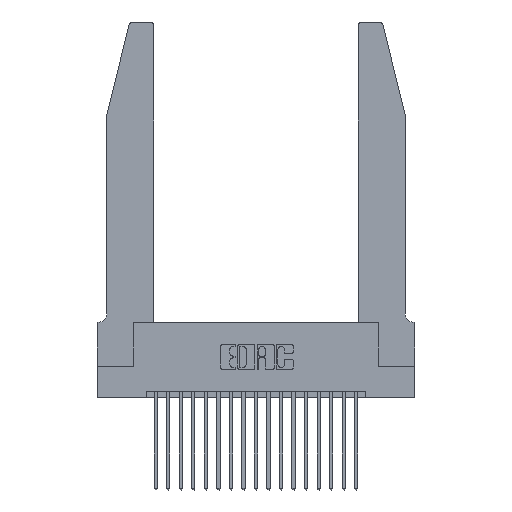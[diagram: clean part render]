
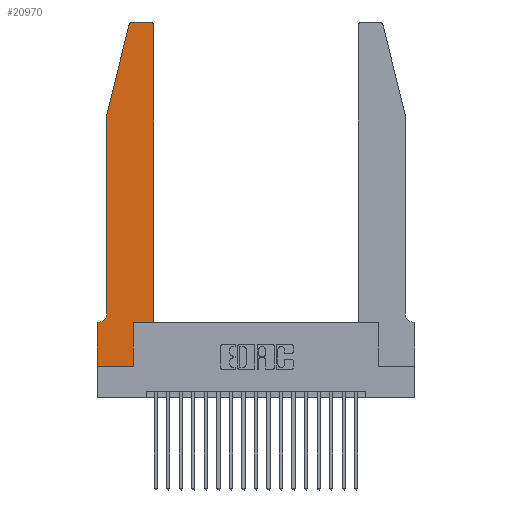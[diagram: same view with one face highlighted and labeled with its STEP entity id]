
A CAD part, top view. The second image highlights one B-rep face of the part: STEP entity #20970.
In plain terms, the highlighted planar face has unit normal (0, 0, 1).
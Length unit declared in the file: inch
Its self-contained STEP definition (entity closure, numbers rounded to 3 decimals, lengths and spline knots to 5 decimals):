
#87 = CARTESIAN_POINT ( 'NONE',  ( 0., 0.35, 0.37 ) ) ;
#249 = LINE ( 'NONE', #2413, #17041 ) ;
#292 = LINE ( 'NONE', #5435, #5316 ) ;
#384 = ORIENTED_EDGE ( 'NONE', *, *, #6104, .T. ) ;
#533 = DIRECTION ( 'NONE',  ( 0., 0., 1. ) ) ;
#713 = VERTEX_POINT ( 'NONE', #17654 ) ;
#732 = EDGE_CURVE ( 'NONE', #21065, #713, #19488, .T. ) ;
#775 = CARTESIAN_POINT ( 'NONE',  ( 0.25487, 2.72718, 0.37 ) ) ;
#1139 = ORIENTED_EDGE ( 'NONE', *, *, #11980, .T. ) ;
#1290 = CARTESIAN_POINT ( 'NONE',  ( 0.0755, 0.35, 0.37 ) ) ;
#1472 = LINE ( 'NONE', #15366, #5440 ) ;
#1486 = CARTESIAN_POINT ( 'NONE',  ( 0.0755, 2., 0.37 ) ) ;
#1848 = VECTOR ( 'NONE', #5260, 39.37008 ) ;
#2008 = CARTESIAN_POINT ( 'NONE',  ( 0., 0.35, 0.37 ) ) ;
#2413 = CARTESIAN_POINT ( 'NONE',  ( 0.4505, 0.35, 0.37 ) ) ;
#3207 = VECTOR ( 'NONE', #8109, 39.37008 ) ;
#3265 = VECTOR ( 'NONE', #12227, 39.37008 ) ;
#3444 = EDGE_LOOP ( 'NONE', ( #13576, #13081, #15457, #16988, #384, #16514, #11763, #8634, #13420, #1139, #20366, #21364 ) ) ;
#3725 = LINE ( 'NONE', #16472, #3207 ) ;
#3901 = EDGE_CURVE ( 'NONE', #11620, #21172, #4140, .T. ) ;
#4140 = LINE ( 'NONE', #1486, #12067 ) ;
#4184 = VERTEX_POINT ( 'NONE', #9055 ) ;
#4361 = VECTOR ( 'NONE', #16434, 39.37008 ) ;
#4559 = CARTESIAN_POINT ( 'NONE',  ( 0.2865, 0., 0.37 ) ) ;
#4640 = VECTOR ( 'NONE', #7286, 39.37008 ) ;
#4713 = EDGE_CURVE ( 'NONE', #20840, #4871, #13579, .T. ) ;
#4871 = VERTEX_POINT ( 'NONE', #17752 ) ;
#4876 = DIRECTION ( 'NONE',  ( 0., -1., 0. ) ) ;
#4877 = DIRECTION ( 'NONE',  ( 1., 0., 0. ) ) ;
#4996 = EDGE_CURVE ( 'NONE', #4184, #20840, #8832, .T. ) ;
#5260 = DIRECTION ( 'NONE',  ( 1., 0., 0. ) ) ;
#5277 = FACE_OUTER_BOUND ( 'NONE', #3444, .T. ) ;
#5316 = VECTOR ( 'NONE', #18728, 39.37008 ) ;
#5435 = CARTESIAN_POINT ( 'NONE',  ( 0.0755, 2., 0.37 ) ) ;
#5440 = VECTOR ( 'NONE', #11983, 39.37008 ) ;
#5601 = CARTESIAN_POINT ( 'NONE',  ( 0., 0., 0.37 ) ) ;
#5630 = CARTESIAN_POINT ( 'NONE',  ( 0.0055, 0.42, 0.37 ) ) ;
#6104 = EDGE_CURVE ( 'NONE', #21172, #4184, #11178, .T. ) ;
#6469 = CARTESIAN_POINT ( 'NONE',  ( 0.0755, 2., 0.37 ) ) ;
#6484 = CIRCLE ( 'NONE', #13476, 0.03 ) ;
#6508 = EDGE_CURVE ( 'NONE', #713, #11640, #16634, .T. ) ;
#7286 = DIRECTION ( 'NONE',  ( 0., -1., 0. ) ) ;
#7318 = DIRECTION ( 'NONE',  ( -1., 0., 0. ) ) ;
#7470 = DIRECTION ( 'NONE',  ( 0., 0., 1. ) ) ;
#8109 = DIRECTION ( 'NONE',  ( 0., 1., 0. ) ) ;
#8634 = ORIENTED_EDGE ( 'NONE', *, *, #20890, .T. ) ;
#8647 = DIRECTION ( 'NONE',  ( 0., 0., 1. ) ) ;
#8808 = VERTEX_POINT ( 'NONE', #4559 ) ;
#8821 = CARTESIAN_POINT ( 'NONE',  ( 0.2605, 2.75, 0.37 ) ) ;
#8832 = LINE ( 'NONE', #1290, #4361 ) ;
#9055 = CARTESIAN_POINT ( 'NONE',  ( 0.0055, 0.35, 0.37 ) ) ;
#9195 = AXIS2_PLACEMENT_3D ( 'NONE', #2008, #533, #12322 ) ;
#9389 = VERTEX_POINT ( 'NONE', #775 ) ;
#10247 = CARTESIAN_POINT ( 'NONE',  ( 0.4505, 0.35, 0.37 ) ) ;
#10838 = LINE ( 'NONE', #16965, #1848 ) ;
#10974 = EDGE_CURVE ( 'NONE', #9389, #11620, #292, .T. ) ;
#11049 = EDGE_CURVE ( 'NONE', #8808, #19170, #3725, .T. ) ;
#11178 = CIRCLE ( 'NONE', #13089, 0.07 ) ;
#11287 = CARTESIAN_POINT ( 'NONE',  ( 0.0755, 0.42, 0.37 ) ) ;
#11620 = VERTEX_POINT ( 'NONE', #6469 ) ;
#11640 = VERTEX_POINT ( 'NONE', #14922 ) ;
#11763 = ORIENTED_EDGE ( 'NONE', *, *, #4713, .T. ) ;
#11980 = EDGE_CURVE ( 'NONE', #19170, #14768, #249, .T. ) ;
#11983 = DIRECTION ( 'NONE',  ( 0., 1., 0. ) ) ;
#12067 = VECTOR ( 'NONE', #4876, 39.37008 ) ;
#12227 = DIRECTION ( 'NONE',  ( -1., 0., 0. ) ) ;
#12322 = DIRECTION ( 'NONE',  ( 1., 0., 0. ) ) ;
#12605 = CARTESIAN_POINT ( 'NONE',  ( 0.4505, 2.72, 0.37 ) ) ;
#13081 = ORIENTED_EDGE ( 'NONE', *, *, #14830, .T. ) ;
#13089 = AXIS2_PLACEMENT_3D ( 'NONE', #5630, #17299, #7318 ) ;
#13420 = ORIENTED_EDGE ( 'NONE', *, *, #11049, .T. ) ;
#13476 = AXIS2_PLACEMENT_3D ( 'NONE', #18577, #8647, #20181 ) ;
#13576 = ORIENTED_EDGE ( 'NONE', *, *, #6508, .T. ) ;
#13579 = LINE ( 'NONE', #5601, #4640 ) ;
#14768 = VERTEX_POINT ( 'NONE', #10247 ) ;
#14830 = EDGE_CURVE ( 'NONE', #11640, #9389, #6484, .T. ) ;
#14831 = EDGE_CURVE ( 'NONE', #14768, #21065, #1472, .T. ) ;
#14922 = CARTESIAN_POINT ( 'NONE',  ( 0.284, 2.75, 0.37 ) ) ;
#15345 = CARTESIAN_POINT ( 'NONE',  ( 0.4205, 2.72, 0.37 ) ) ;
#15366 = CARTESIAN_POINT ( 'NONE',  ( 0.4505, 0.35, 0.37 ) ) ;
#15457 = ORIENTED_EDGE ( 'NONE', *, *, #10974, .T. ) ;
#16434 = DIRECTION ( 'NONE',  ( -1., 0., 0. ) ) ;
#16472 = CARTESIAN_POINT ( 'NONE',  ( 0.2865, 0.35, 0.37 ) ) ;
#16514 = ORIENTED_EDGE ( 'NONE', *, *, #4996, .T. ) ;
#16634 = LINE ( 'NONE', #8821, #3265 ) ;
#16965 = CARTESIAN_POINT ( 'NONE',  ( 0., 0., 0.37 ) ) ;
#16988 = ORIENTED_EDGE ( 'NONE', *, *, #3901, .T. ) ;
#17041 = VECTOR ( 'NONE', #20664, 39.37008 ) ;
#17299 = DIRECTION ( 'NONE',  ( 0., 0., -1. ) ) ;
#17654 = CARTESIAN_POINT ( 'NONE',  ( 0.4205, 2.75, 0.37 ) ) ;
#17742 = AXIS2_PLACEMENT_3D ( 'NONE', #15345, #7470, #4877 ) ;
#17752 = CARTESIAN_POINT ( 'NONE',  ( 0., 0., 0.37 ) ) ;
#18577 = CARTESIAN_POINT ( 'NONE',  ( 0.284, 2.72, 0.37 ) ) ;
#18728 = DIRECTION ( 'NONE',  ( -0.239, -0.971, 0. ) ) ;
#19170 = VERTEX_POINT ( 'NONE', #19652 ) ;
#19488 = CIRCLE ( 'NONE', #17742, 0.03 ) ;
#19652 = CARTESIAN_POINT ( 'NONE',  ( 0.2865, 0.35, 0.37 ) ) ;
#20181 = DIRECTION ( 'NONE',  ( 1., 0., 0. ) ) ;
#20366 = ORIENTED_EDGE ( 'NONE', *, *, #14831, .T. ) ;
#20429 = PLANE ( 'NONE',  #9195 ) ;
#20664 = DIRECTION ( 'NONE',  ( 1., 0., 0. ) ) ;
#20840 = VERTEX_POINT ( 'NONE', #87 ) ;
#20890 = EDGE_CURVE ( 'NONE', #4871, #8808, #10838, .T. ) ;
#20970 = ADVANCED_FACE ( 'NONE', ( #5277 ), #20429, .T. ) ;
#21065 = VERTEX_POINT ( 'NONE', #12605 ) ;
#21172 = VERTEX_POINT ( 'NONE', #11287 ) ;
#21364 = ORIENTED_EDGE ( 'NONE', *, *, #732, .T. ) ;
